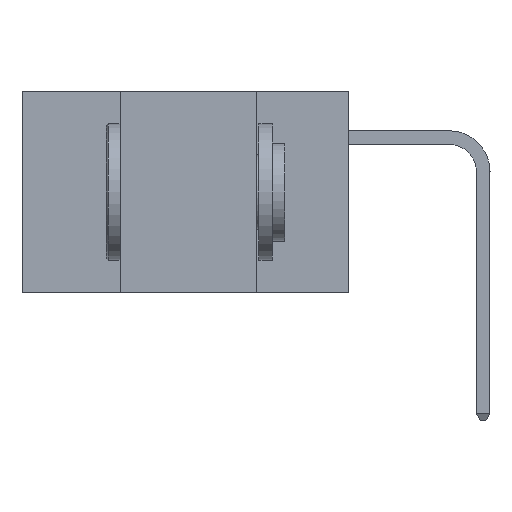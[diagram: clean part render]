
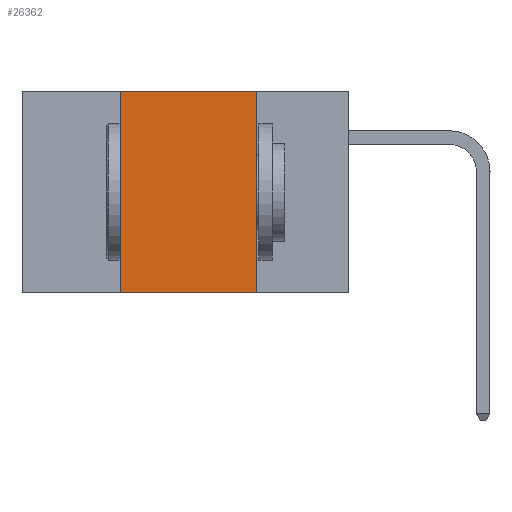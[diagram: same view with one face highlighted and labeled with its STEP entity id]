
A CAD part, left-side view. The second image highlights one B-rep face of the part: STEP entity #26362.
In plain terms, the highlighted planar face has unit normal (-1, 0, 0).
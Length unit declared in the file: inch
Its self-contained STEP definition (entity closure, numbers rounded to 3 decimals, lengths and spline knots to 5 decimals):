
#2204 = CARTESIAN_POINT ( 'NONE',  ( 0., 0.6, 0. ) ) ;
#2345 = PLANE ( 'NONE',  #37671 ) ;
#3712 = DIRECTION ( 'NONE',  ( 0., -1., 0. ) ) ;
#3789 = ORIENTED_EDGE ( 'NONE', *, *, #34441, .F. ) ;
#7661 = CARTESIAN_POINT ( 'NONE',  ( 0., 0.42, 0. ) ) ;
#7925 = ORIENTED_EDGE ( 'NONE', *, *, #27649, .T. ) ;
#9709 = VERTEX_POINT ( 'NONE', #25280 ) ;
#11284 = DIRECTION ( 'NONE',  ( 1., 0., 0. ) ) ;
#13470 = VECTOR ( 'NONE', #23644, 39.37008 ) ;
#14557 = CARTESIAN_POINT ( 'NONE',  ( 0., 0.6, -0.37 ) ) ;
#19319 = VECTOR ( 'NONE', #31392, 39.37008 ) ;
#19552 = VECTOR ( 'NONE', #34828, 39.37008 ) ;
#19700 = VECTOR ( 'NONE', #3712, 39.37008 ) ;
#20390 = ORIENTED_EDGE ( 'NONE', *, *, #37293, .F. ) ;
#20484 = LINE ( 'NONE', #14557, #19552 ) ;
#23644 = DIRECTION ( 'NONE',  ( 0., 0., -1. ) ) ;
#25280 = CARTESIAN_POINT ( 'NONE',  ( 0., 0.42, 0. ) ) ;
#26272 = ORIENTED_EDGE ( 'NONE', *, *, #33439, .F. ) ;
#26362 = ADVANCED_FACE ( 'NONE', ( #31919 ), #2345, .F. ) ;
#27401 = LINE ( 'NONE', #35706, #19700 ) ;
#27527 = EDGE_LOOP ( 'NONE', ( #20390, #3789, #26272, #7925 ) ) ;
#27649 = EDGE_CURVE ( 'NONE', #34851, #34997, #20484, .T. ) ;
#29746 = CARTESIAN_POINT ( 'NONE',  ( 0., 0.42, -0.37 ) ) ;
#31392 = DIRECTION ( 'NONE',  ( 0., 0., 1. ) ) ;
#31665 = DIRECTION ( 'NONE',  ( 0., 0., -1. ) ) ;
#31919 = FACE_OUTER_BOUND ( 'NONE', #27527, .T. ) ;
#33439 = EDGE_CURVE ( 'NONE', #34851, #9709, #34682, .T. ) ;
#34441 = EDGE_CURVE ( 'NONE', #9709, #35642, #27401, .T. ) ;
#34682 = LINE ( 'NONE', #7661, #19319 ) ;
#34828 = DIRECTION ( 'NONE',  ( 0., -1., 0. ) ) ;
#34851 = VERTEX_POINT ( 'NONE', #29746 ) ;
#34997 = VERTEX_POINT ( 'NONE', #36133 ) ;
#35080 = CARTESIAN_POINT ( 'NONE',  ( 0., 0.17, 0. ) ) ;
#35642 = VERTEX_POINT ( 'NONE', #36202 ) ;
#35696 = LINE ( 'NONE', #35080, #13470 ) ;
#35706 = CARTESIAN_POINT ( 'NONE',  ( 0., 0.6, 0. ) ) ;
#36133 = CARTESIAN_POINT ( 'NONE',  ( 0., 0.17, -0.37 ) ) ;
#36202 = CARTESIAN_POINT ( 'NONE',  ( 0., 0.17, 0. ) ) ;
#37293 = EDGE_CURVE ( 'NONE', #35642, #34997, #35696, .T. ) ;
#37671 = AXIS2_PLACEMENT_3D ( 'NONE', #2204, #11284, #31665 ) ;
